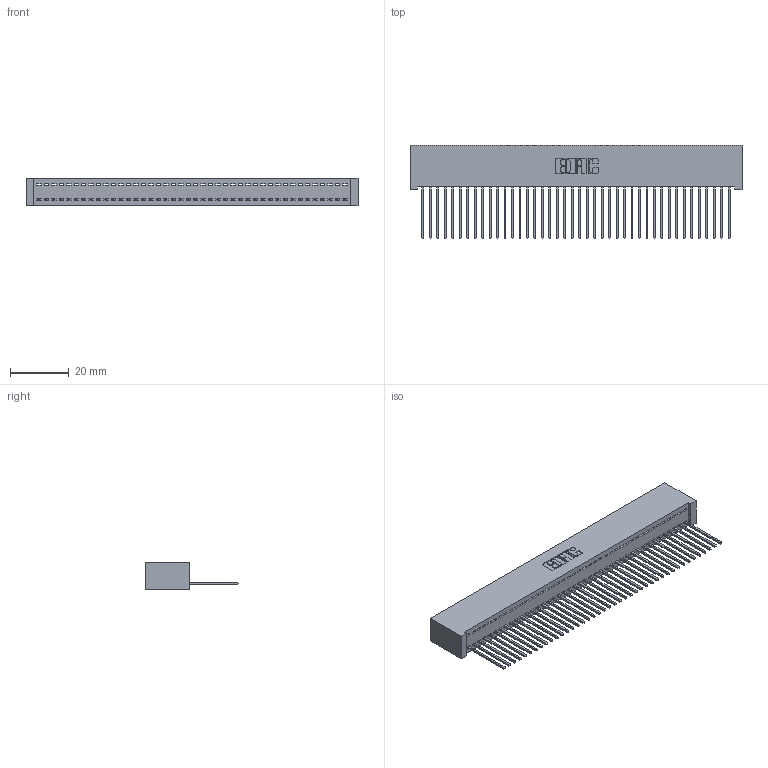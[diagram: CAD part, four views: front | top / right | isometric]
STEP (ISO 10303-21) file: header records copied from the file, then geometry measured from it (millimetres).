
FILE_DESCRIPTION (( 'STEP AP203' ), '1' );
FILE_NAME ('392-042-542-101.STEP', '2019-10-07T21:10:55', ( '' ), ( '' ), 'SwSTEP 2.0', 'SolidWorks 2016', '' );
FILE_SCHEMA (( 'CONFIG_CONTROL_DESIGN' ));
Length unit declared in the file: inch
Products named in the file (3): 342 Part_Lugless; 345-292-001_345-293-142; 392-042-542-101
Assembly tree (43 placements, depth 2):
  392-042-542-101
    342 Part_Lugless
    345-292-001_345-293-142  x42
Bounding box: 112.93 x 31.63 x 9.4 mm (x, y, z)
Volume: 10404 mm3; surface area: 16171 mm2
Topology: 43 solids, 43 shells, 2538 faces, 7667 edges, 5054 vertices
Faces by surface type: plane 1826, cylinder 712
Entity records: 25285 total; most frequent: CARTESIAN_POINT 4368, ORIENTED_EDGE 4346, DIRECTION 3677, EDGE_CURVE 2173, VECTOR 2053, LINE 2053, VERTEX_POINT 1446, AXIS2_PLACEMENT_3D 812
